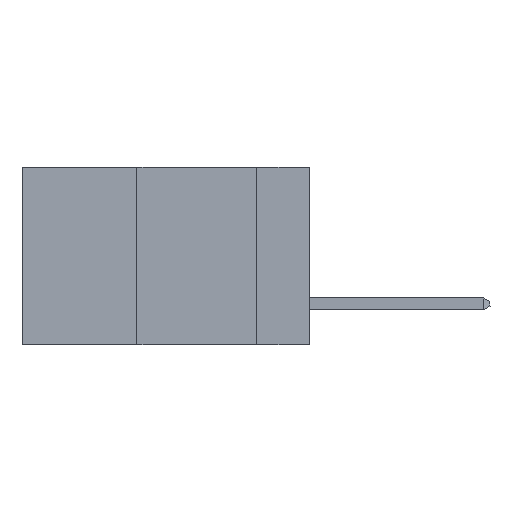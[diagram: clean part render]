
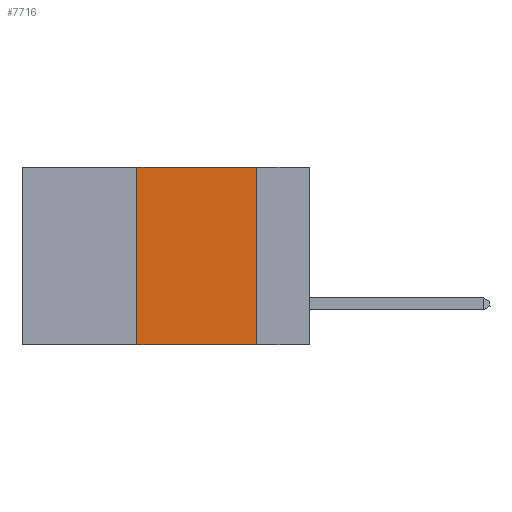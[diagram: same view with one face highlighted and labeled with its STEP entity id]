
A CAD part, left-side view. The second image highlights one B-rep face of the part: STEP entity #7716.
In plain terms, the highlighted planar face has unit normal (-1, 0, 0).
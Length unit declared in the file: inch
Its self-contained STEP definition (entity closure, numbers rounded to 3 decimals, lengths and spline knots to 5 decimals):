
#693 = VERTEX_POINT ( 'NONE', #11174 ) ;
#752 = ORIENTED_EDGE ( 'NONE', *, *, #1907, .F. ) ;
#1305 = EDGE_CURVE ( 'NONE', #3713, #7295, #6042, .T. ) ;
#1510 = VECTOR ( 'NONE', #13947, 39.37008 ) ;
#1863 = PLANE ( 'NONE',  #2156 ) ;
#1905 = EDGE_CURVE ( 'NONE', #7295, #693, #8558, .T. ) ;
#1907 = EDGE_CURVE ( 'NONE', #7293, #3713, #10829, .T. ) ;
#1909 = EDGE_CURVE ( 'NONE', #7293, #693, #1944, .T. ) ;
#1944 = LINE ( 'NONE', #13991, #10502 ) ;
#2156 = AXIS2_PLACEMENT_3D ( 'NONE', #4451, #12243, #5627 ) ;
#3242 = VECTOR ( 'NONE', #4753, 39.37008 ) ;
#3713 = VERTEX_POINT ( 'NONE', #8478 ) ;
#4451 = CARTESIAN_POINT ( 'NONE',  ( 0., 0.6, 0. ) ) ;
#4541 = ORIENTED_EDGE ( 'NONE', *, *, #1305, .F. ) ;
#4753 = DIRECTION ( 'NONE',  ( 0., -1., 0. ) ) ;
#5576 = CARTESIAN_POINT ( 'NONE',  ( 0., 0.6, 0. ) ) ;
#5627 = DIRECTION ( 'NONE',  ( 0., 0., -1. ) ) ;
#5787 = ORIENTED_EDGE ( 'NONE', *, *, #1905, .F. ) ;
#6042 = LINE ( 'NONE', #5576, #3242 ) ;
#6094 = CARTESIAN_POINT ( 'NONE',  ( 0., 0.11, 0. ) ) ;
#7293 = VERTEX_POINT ( 'NONE', #11578 ) ;
#7295 = VERTEX_POINT ( 'NONE', #6094 ) ;
#7716 = ADVANCED_FACE ( 'NONE', ( #13104 ), #1863, .F. ) ;
#7896 = VECTOR ( 'NONE', #13686, 39.37008 ) ;
#7918 = ORIENTED_EDGE ( 'NONE', *, *, #1909, .T. ) ;
#8478 = CARTESIAN_POINT ( 'NONE',  ( 0., 0.36, 0. ) ) ;
#8558 = LINE ( 'NONE', #13698, #7896 ) ;
#10502 = VECTOR ( 'NONE', #13830, 39.37008 ) ;
#10829 = LINE ( 'NONE', #13599, #1510 ) ;
#11174 = CARTESIAN_POINT ( 'NONE',  ( 0., 0.11, -0.37 ) ) ;
#11578 = CARTESIAN_POINT ( 'NONE',  ( 0., 0.36, -0.37 ) ) ;
#12243 = DIRECTION ( 'NONE',  ( 1., 0., 0. ) ) ;
#13104 = FACE_OUTER_BOUND ( 'NONE', #13313, .T. ) ;
#13313 = EDGE_LOOP ( 'NONE', ( #5787, #4541, #752, #7918 ) ) ;
#13599 = CARTESIAN_POINT ( 'NONE',  ( 0., 0.36, 0. ) ) ;
#13686 = DIRECTION ( 'NONE',  ( 0., 0., -1. ) ) ;
#13698 = CARTESIAN_POINT ( 'NONE',  ( 0., 0.11, 0. ) ) ;
#13830 = DIRECTION ( 'NONE',  ( 0., -1., 0. ) ) ;
#13947 = DIRECTION ( 'NONE',  ( 0., 0., 1. ) ) ;
#13991 = CARTESIAN_POINT ( 'NONE',  ( 0., 0.6, -0.37 ) ) ;
